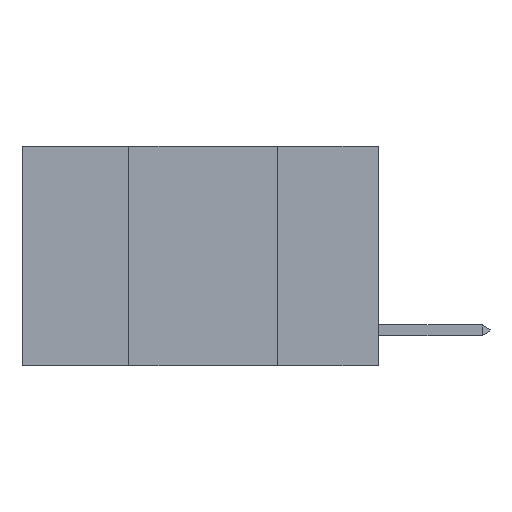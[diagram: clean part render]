
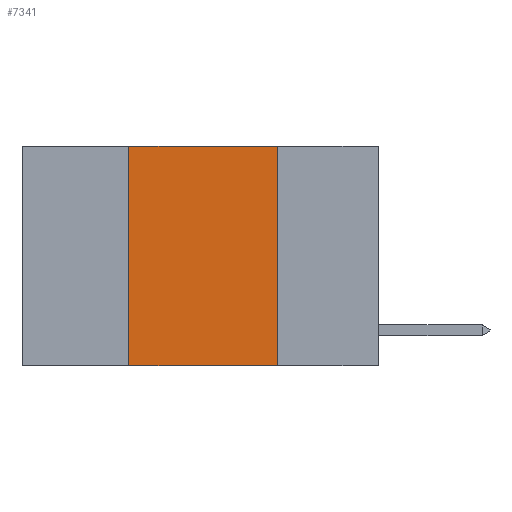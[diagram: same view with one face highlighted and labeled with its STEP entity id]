
A CAD part, left-side view. The second image highlights one B-rep face of the part: STEP entity #7341.
In plain terms, the highlighted planar face has unit normal (-1, 0, 0).
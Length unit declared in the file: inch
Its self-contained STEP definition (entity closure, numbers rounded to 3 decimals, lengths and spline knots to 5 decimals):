
#195 = PLANE ( 'NONE',  #13796 ) ;
#1711 = VECTOR ( 'NONE', #16462, 39.37008 ) ;
#2086 = DIRECTION ( 'NONE',  ( 1., 0., 0. ) ) ;
#2730 = VERTEX_POINT ( 'NONE', #8663 ) ;
#4346 = CARTESIAN_POINT ( 'NONE',  ( 0., 0.42, 0. ) ) ;
#4581 = ORIENTED_EDGE ( 'NONE', *, *, #20606, .T. ) ;
#5248 = LINE ( 'NONE', #17480, #10278 ) ;
#5801 = CARTESIAN_POINT ( 'NONE',  ( 0., 0.6, 0. ) ) ;
#6268 = DIRECTION ( 'NONE',  ( 0., 0., 1. ) ) ;
#6700 = ORIENTED_EDGE ( 'NONE', *, *, #14548, .F. ) ;
#7341 = ADVANCED_FACE ( 'NONE', ( #18420 ), #195, .F. ) ;
#8549 = VECTOR ( 'NONE', #17403, 39.37008 ) ;
#8663 = CARTESIAN_POINT ( 'NONE',  ( 0., 0.42, 0. ) ) ;
#10278 = VECTOR ( 'NONE', #21088, 39.37008 ) ;
#12439 = EDGE_LOOP ( 'NONE', ( #6700, #19682, #16307, #4581 ) ) ;
#12924 = LINE ( 'NONE', #21722, #1711 ) ;
#13796 = AXIS2_PLACEMENT_3D ( 'NONE', #5801, #2086, #15210 ) ;
#14548 = EDGE_CURVE ( 'NONE', #15325, #19619, #5248, .T. ) ;
#15210 = DIRECTION ( 'NONE',  ( 0., 0., -1. ) ) ;
#15325 = VERTEX_POINT ( 'NONE', #16028 ) ;
#15571 = CARTESIAN_POINT ( 'NONE',  ( 0., 0.6, -0.37 ) ) ;
#16028 = CARTESIAN_POINT ( 'NONE',  ( 0., 0.17, 0. ) ) ;
#16307 = ORIENTED_EDGE ( 'NONE', *, *, #16972, .F. ) ;
#16462 = DIRECTION ( 'NONE',  ( 0., -1., 0. ) ) ;
#16972 = EDGE_CURVE ( 'NONE', #21146, #2730, #19319, .T. ) ;
#17403 = DIRECTION ( 'NONE',  ( 0., -1., 0. ) ) ;
#17480 = CARTESIAN_POINT ( 'NONE',  ( 0., 0.17, 0. ) ) ;
#18144 = CARTESIAN_POINT ( 'NONE',  ( 0., 0.17, -0.37 ) ) ;
#18196 = VECTOR ( 'NONE', #6268, 39.37008 ) ;
#18420 = FACE_OUTER_BOUND ( 'NONE', #12439, .T. ) ;
#19319 = LINE ( 'NONE', #4346, #18196 ) ;
#19331 = CARTESIAN_POINT ( 'NONE',  ( 0., 0.42, -0.37 ) ) ;
#19619 = VERTEX_POINT ( 'NONE', #18144 ) ;
#19682 = ORIENTED_EDGE ( 'NONE', *, *, #21923, .F. ) ;
#20606 = EDGE_CURVE ( 'NONE', #21146, #19619, #23671, .T. ) ;
#21088 = DIRECTION ( 'NONE',  ( 0., 0., -1. ) ) ;
#21146 = VERTEX_POINT ( 'NONE', #19331 ) ;
#21722 = CARTESIAN_POINT ( 'NONE',  ( 0., 0.6, 0. ) ) ;
#21923 = EDGE_CURVE ( 'NONE', #2730, #15325, #12924, .T. ) ;
#23671 = LINE ( 'NONE', #15571, #8549 ) ;
